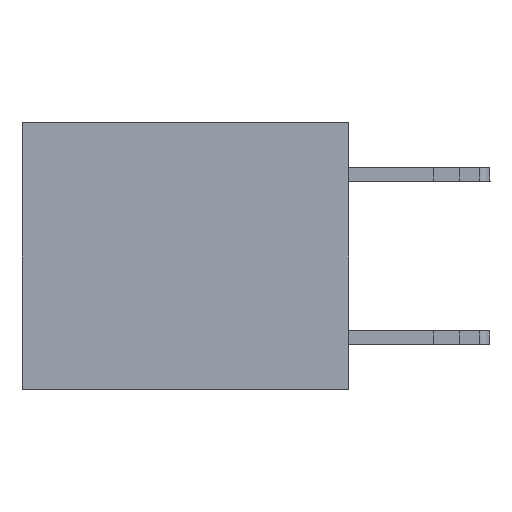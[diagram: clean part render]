
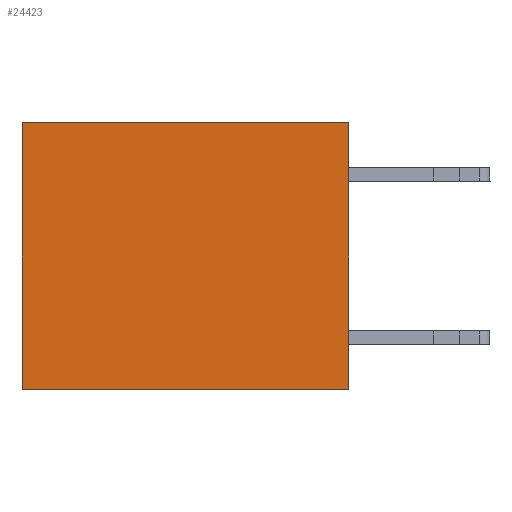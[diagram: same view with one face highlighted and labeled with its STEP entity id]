
A CAD part, left-side view. The second image highlights one B-rep face of the part: STEP entity #24423.
In plain terms, the highlighted planar face has unit normal (-1, 0, 0).
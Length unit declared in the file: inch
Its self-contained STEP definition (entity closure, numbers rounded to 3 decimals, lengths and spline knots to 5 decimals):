
#422 = EDGE_CURVE ( 'NONE', #19964, #20133, #26529, .T. ) ;
#528 = LINE ( 'NONE', #21154, #22117 ) ;
#1434 = VECTOR ( 'NONE', #11796, 39.37008 ) ;
#2843 = DIRECTION ( 'NONE',  ( 0., 0., -1. ) ) ;
#2930 = CARTESIAN_POINT ( 'NONE',  ( 0.3165, 0., -0.49 ) ) ;
#3026 = CARTESIAN_POINT ( 'NONE',  ( 0.3165, 0.6, -0.49 ) ) ;
#3702 = DIRECTION ( 'NONE',  ( 1., 0., 0. ) ) ;
#3802 = PLANE ( 'NONE',  #27347 ) ;
#7067 = EDGE_CURVE ( 'NONE', #11165, #19964, #15961, .T. ) ;
#8295 = CARTESIAN_POINT ( 'NONE',  ( 0.3165, 0., -0.49 ) ) ;
#9917 = VECTOR ( 'NONE', #19082, 39.37008 ) ;
#10696 = CARTESIAN_POINT ( 'NONE',  ( 0.3165, 0., -0.49 ) ) ;
#10782 = DIRECTION ( 'NONE',  ( 0., 0., -1. ) ) ;
#11165 = VERTEX_POINT ( 'NONE', #25986 ) ;
#11796 = DIRECTION ( 'NONE',  ( 0., 1., 0. ) ) ;
#12388 = CARTESIAN_POINT ( 'NONE',  ( 0.3165, 0.6, 0. ) ) ;
#12650 = ORIENTED_EDGE ( 'NONE', *, *, #28152, .F. ) ;
#15333 = ORIENTED_EDGE ( 'NONE', *, *, #23911, .F. ) ;
#15719 = VERTEX_POINT ( 'NONE', #8295 ) ;
#15961 = LINE ( 'NONE', #17021, #9917 ) ;
#17021 = CARTESIAN_POINT ( 'NONE',  ( 0.3165, 0., 0. ) ) ;
#18616 = ORIENTED_EDGE ( 'NONE', *, *, #422, .T. ) ;
#18994 = DIRECTION ( 'NONE',  ( 0., 0., -1. ) ) ;
#19082 = DIRECTION ( 'NONE',  ( 0., 1., 0. ) ) ;
#19964 = VERTEX_POINT ( 'NONE', #12388 ) ;
#20133 = VERTEX_POINT ( 'NONE', #22275 ) ;
#20810 = FACE_OUTER_BOUND ( 'NONE', #23235, .T. ) ;
#21154 = CARTESIAN_POINT ( 'NONE',  ( 0.3165, 0., -0.49 ) ) ;
#22041 = ORIENTED_EDGE ( 'NONE', *, *, #7067, .T. ) ;
#22117 = VECTOR ( 'NONE', #18994, 39.37008 ) ;
#22275 = CARTESIAN_POINT ( 'NONE',  ( 0.3165, 0.6, -0.49 ) ) ;
#23235 = EDGE_LOOP ( 'NONE', ( #18616, #15333, #12650, #22041 ) ) ;
#23911 = EDGE_CURVE ( 'NONE', #15719, #20133, #28299, .T. ) ;
#24423 = ADVANCED_FACE ( 'NONE', ( #20810 ), #3802, .F. ) ;
#25100 = VECTOR ( 'NONE', #2843, 39.37008 ) ;
#25986 = CARTESIAN_POINT ( 'NONE',  ( 0.3165, 0., 0. ) ) ;
#26529 = LINE ( 'NONE', #3026, #25100 ) ;
#27347 = AXIS2_PLACEMENT_3D ( 'NONE', #10696, #3702, #10782 ) ;
#28152 = EDGE_CURVE ( 'NONE', #11165, #15719, #528, .T. ) ;
#28299 = LINE ( 'NONE', #2930, #1434 ) ;
